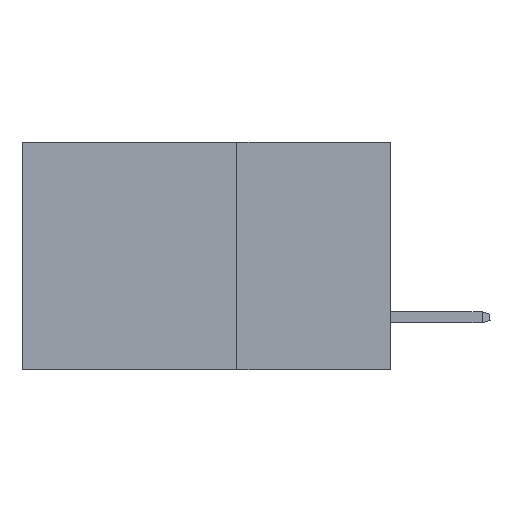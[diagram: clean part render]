
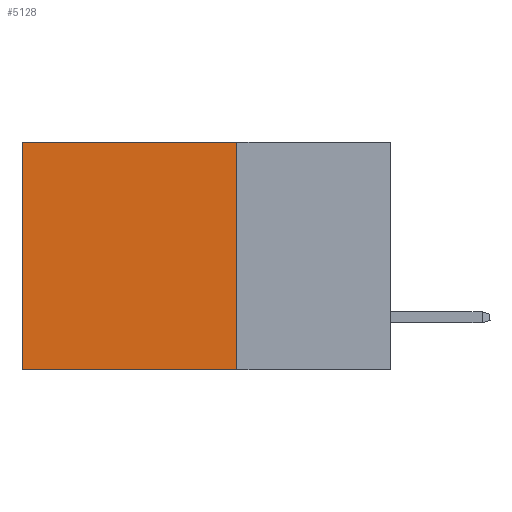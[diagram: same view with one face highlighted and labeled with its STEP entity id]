
A CAD part, left-side view. The second image highlights one B-rep face of the part: STEP entity #5128.
In plain terms, the highlighted planar face has unit normal (-1, 0, 0).
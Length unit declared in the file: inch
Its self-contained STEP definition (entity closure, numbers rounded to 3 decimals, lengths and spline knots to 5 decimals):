
#527 = CARTESIAN_POINT ( 'NONE',  ( 0.2875, 0.6, 0. ) ) ;
#551 = DIRECTION ( 'NONE',  ( 1., 0., 0. ) ) ;
#681 = VECTOR ( 'NONE', #2998, 39.37008 ) ;
#1343 = DIRECTION ( 'NONE',  ( 0., 1., 0. ) ) ;
#1450 = LINE ( 'NONE', #2921, #681 ) ;
#2182 = DIRECTION ( 'NONE',  ( 0., 0., -1. ) ) ;
#2280 = CARTESIAN_POINT ( 'NONE',  ( 0.2875, 0.25, 0. ) ) ;
#2431 = CARTESIAN_POINT ( 'NONE',  ( 0.2875, 0.25, -0.37 ) ) ;
#2626 = ORIENTED_EDGE ( 'NONE', *, *, #9842, .F. ) ;
#2921 = CARTESIAN_POINT ( 'NONE',  ( 0.2875, 0.6, 0. ) ) ;
#2998 = DIRECTION ( 'NONE',  ( 0., 0., -1. ) ) ;
#3042 = LINE ( 'NONE', #3889, #10065 ) ;
#3156 = FACE_OUTER_BOUND ( 'NONE', #6232, .T. ) ;
#3318 = VECTOR ( 'NONE', #3512, 39.37008 ) ;
#3512 = DIRECTION ( 'NONE',  ( 0., 1., 0. ) ) ;
#3889 = CARTESIAN_POINT ( 'NONE',  ( 0.2875, 0.25, 0. ) ) ;
#4214 = AXIS2_PLACEMENT_3D ( 'NONE', #7965, #551, #2182 ) ;
#4477 = VECTOR ( 'NONE', #8781, 39.37008 ) ;
#4549 = EDGE_CURVE ( 'NONE', #6802, #9253, #3042, .T. ) ;
#4584 = EDGE_CURVE ( 'NONE', #6802, #8805, #8395, .T. ) ;
#4887 = CARTESIAN_POINT ( 'NONE',  ( 0.2875, 0.6, -0.37 ) ) ;
#5128 = ADVANCED_FACE ( 'NONE', ( #3156 ), #7116, .F. ) ;
#5510 = ORIENTED_EDGE ( 'NONE', *, *, #5606, .T. ) ;
#5606 = EDGE_CURVE ( 'NONE', #9253, #10368, #1450, .T. ) ;
#6232 = EDGE_LOOP ( 'NONE', ( #5510, #2626, #9627, #7004 ) ) ;
#6802 = VERTEX_POINT ( 'NONE', #2280 ) ;
#7004 = ORIENTED_EDGE ( 'NONE', *, *, #4549, .T. ) ;
#7116 = PLANE ( 'NONE',  #4214 ) ;
#7131 = CARTESIAN_POINT ( 'NONE',  ( 0.2875, 0.25, 0. ) ) ;
#7965 = CARTESIAN_POINT ( 'NONE',  ( 0.2875, 0.25, 0. ) ) ;
#8395 = LINE ( 'NONE', #7131, #4477 ) ;
#8781 = DIRECTION ( 'NONE',  ( 0., 0., -1. ) ) ;
#8805 = VERTEX_POINT ( 'NONE', #9885 ) ;
#9253 = VERTEX_POINT ( 'NONE', #527 ) ;
#9627 = ORIENTED_EDGE ( 'NONE', *, *, #4584, .F. ) ;
#9700 = LINE ( 'NONE', #2431, #3318 ) ;
#9842 = EDGE_CURVE ( 'NONE', #8805, #10368, #9700, .T. ) ;
#9885 = CARTESIAN_POINT ( 'NONE',  ( 0.2875, 0.25, -0.37 ) ) ;
#10065 = VECTOR ( 'NONE', #1343, 39.37008 ) ;
#10368 = VERTEX_POINT ( 'NONE', #4887 ) ;
